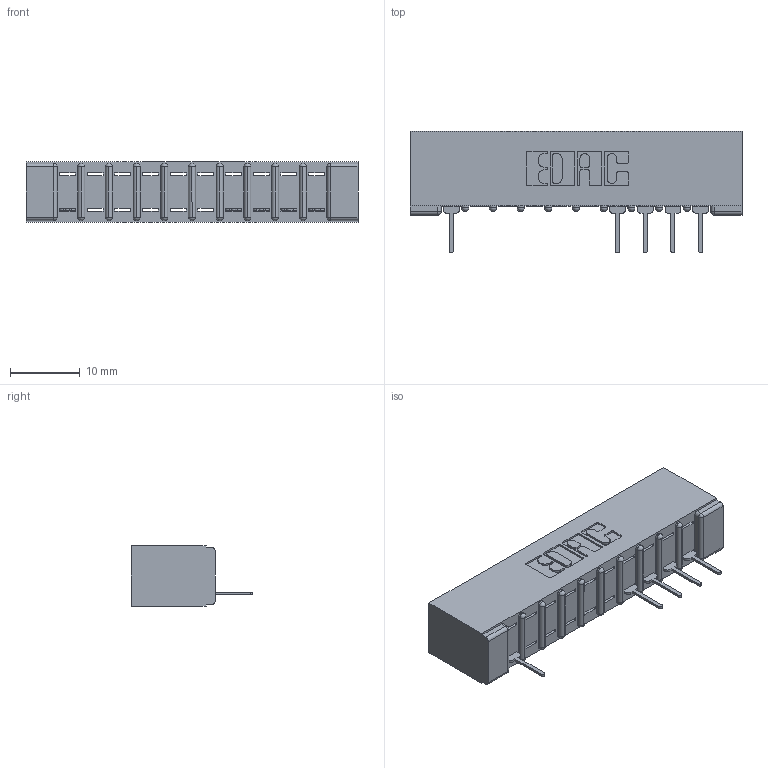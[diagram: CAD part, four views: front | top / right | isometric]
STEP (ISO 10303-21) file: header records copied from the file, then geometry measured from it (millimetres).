
FILE_DESCRIPTION (( 'STEP AP203' ), '1' );
FILE_NAME ('357-010-531-101.STEP', '2018-08-07T02:35:56', ( '' ), ( '' ), 'SwSTEP 2.0', 'SolidWorks 2016', '' );
FILE_SCHEMA (( 'CONFIG_CONTROL_DESIGN' ));
Length unit declared in the file: inch
Products named in the file (3): 307-290-001_531; 357-010-531-101; 307 Part_No Mounting Lugs
Assembly tree (6 placements, depth 2):
  357-010-531-101
    307 Part_No Mounting Lugs
    307-290-001_531  x5
Bounding box: 47.5 x 17.42 x 8.71 mm (x, y, z)
Volume: 3145.7 mm3; surface area: 4247.1 mm2
Topology: 6 solids, 6 shells, 501 faces, 1429 edges, 914 vertices
Faces by surface type: plane 311, cylinder 168, sphere 22
Entity records: 12048 total; most frequent: CARTESIAN_POINT 2039, ORIENTED_EDGE 2030, DIRECTION 1995, EDGE_CURVE 1015, VECTOR 767, LINE 767, VERTEX_POINT 658, AXIS2_PLACEMENT_3D 614
